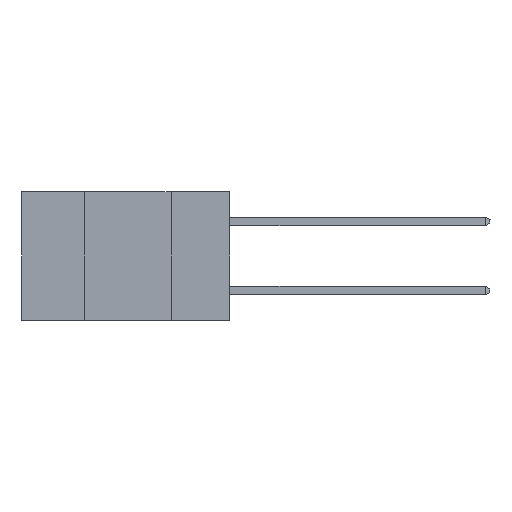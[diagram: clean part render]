
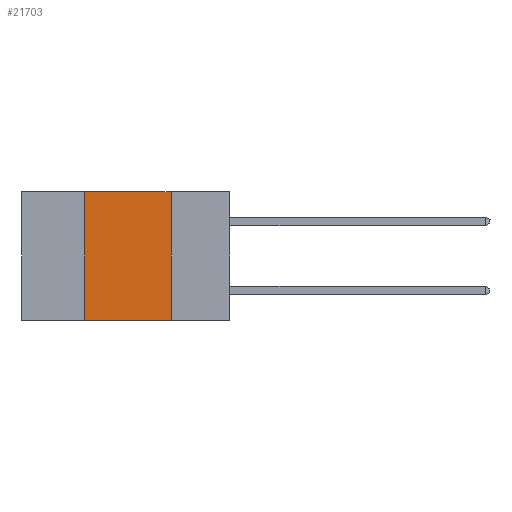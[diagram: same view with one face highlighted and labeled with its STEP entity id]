
A CAD part, left-side view. The second image highlights one B-rep face of the part: STEP entity #21703.
In plain terms, the highlighted planar face has unit normal (-1, 0, 0).
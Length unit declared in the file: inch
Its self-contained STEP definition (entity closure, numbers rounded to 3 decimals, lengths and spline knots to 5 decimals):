
#1346 = DIRECTION ( 'NONE',  ( 0., -1., 0. ) ) ;
#2000 = DIRECTION ( 'NONE',  ( 0., -1., 0. ) ) ;
#2784 = EDGE_CURVE ( 'NONE', #25444, #7408, #6037, .T. ) ;
#2941 = ORIENTED_EDGE ( 'NONE', *, *, #21239, .F. ) ;
#4538 = VERTEX_POINT ( 'NONE', #24618 ) ;
#6037 = LINE ( 'NONE', #14405, #17383 ) ;
#6505 = LINE ( 'NONE', #6885, #25031 ) ;
#6885 = CARTESIAN_POINT ( 'NONE',  ( 0., 0.6, 0. ) ) ;
#7408 = VERTEX_POINT ( 'NONE', #18142 ) ;
#8493 = CARTESIAN_POINT ( 'NONE',  ( 0., 0.17, 0. ) ) ;
#8999 = FACE_OUTER_BOUND ( 'NONE', #20987, .T. ) ;
#9509 = DIRECTION ( 'NONE',  ( 1., 0., 0. ) ) ;
#10547 = EDGE_CURVE ( 'NONE', #4538, #25444, #6505, .T. ) ;
#11852 = CARTESIAN_POINT ( 'NONE',  ( 0., 0.6, 0. ) ) ;
#12340 = DIRECTION ( 'NONE',  ( 0., 0., -1. ) ) ;
#12420 = VECTOR ( 'NONE', #1346, 39.37008 ) ;
#12831 = DIRECTION ( 'NONE',  ( 0., 0., 1. ) ) ;
#13786 = AXIS2_PLACEMENT_3D ( 'NONE', #11852, #9509, #26384 ) ;
#14405 = CARTESIAN_POINT ( 'NONE',  ( 0., 0.17, 0. ) ) ;
#14765 = EDGE_CURVE ( 'NONE', #21719, #7408, #25249, .T. ) ;
#15840 = ORIENTED_EDGE ( 'NONE', *, *, #10547, .F. ) ;
#17383 = VECTOR ( 'NONE', #12340, 39.37008 ) ;
#17568 = CARTESIAN_POINT ( 'NONE',  ( 0., 0.42, 0. ) ) ;
#18142 = CARTESIAN_POINT ( 'NONE',  ( 0., 0.17, -0.37 ) ) ;
#20349 = VECTOR ( 'NONE', #12831, 39.37008 ) ;
#20987 = EDGE_LOOP ( 'NONE', ( #27222, #15840, #2941, #27120 ) ) ;
#21239 = EDGE_CURVE ( 'NONE', #21719, #4538, #28215, .T. ) ;
#21703 = ADVANCED_FACE ( 'NONE', ( #8999 ), #23970, .F. ) ;
#21719 = VERTEX_POINT ( 'NONE', #31117 ) ;
#23970 = PLANE ( 'NONE',  #13786 ) ;
#24618 = CARTESIAN_POINT ( 'NONE',  ( 0., 0.42, 0. ) ) ;
#25031 = VECTOR ( 'NONE', #2000, 39.37008 ) ;
#25249 = LINE ( 'NONE', #30212, #12420 ) ;
#25444 = VERTEX_POINT ( 'NONE', #8493 ) ;
#26384 = DIRECTION ( 'NONE',  ( 0., 0., -1. ) ) ;
#27120 = ORIENTED_EDGE ( 'NONE', *, *, #14765, .T. ) ;
#27222 = ORIENTED_EDGE ( 'NONE', *, *, #2784, .F. ) ;
#28215 = LINE ( 'NONE', #17568, #20349 ) ;
#30212 = CARTESIAN_POINT ( 'NONE',  ( 0., 0.6, -0.37 ) ) ;
#31117 = CARTESIAN_POINT ( 'NONE',  ( 0., 0.42, -0.37 ) ) ;
